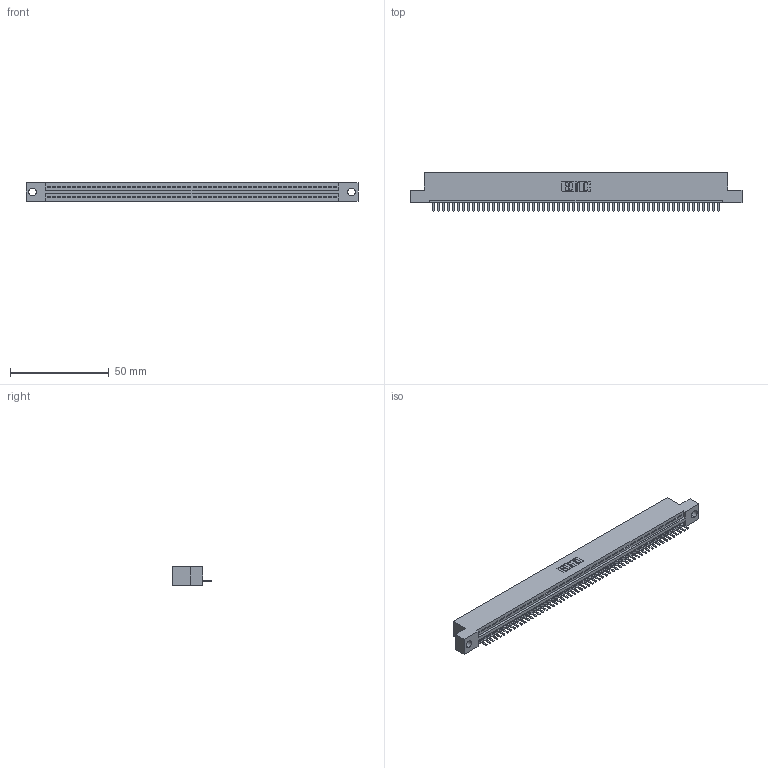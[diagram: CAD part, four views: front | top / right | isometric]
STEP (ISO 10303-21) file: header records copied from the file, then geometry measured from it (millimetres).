
FILE_DESCRIPTION (( 'STEP AP203' ), '1' );
FILE_NAME ('395-058-520-104.STEP', '2018-11-22T23:56:21', ( '' ), ( '' ), 'SwSTEP 2.0', 'SolidWorks 2016', '' );
FILE_SCHEMA (( 'CONFIG_CONTROL_DESIGN' ));
Length unit declared in the file: inch
Products named in the file (3): 345-292-001_345-293-120; 345 Part_Flush Mounting Lugs - 0.156 Dia-TH; 395-058-520-104
Assembly tree (59 placements, depth 2):
  395-058-520-104
    345 Part_Flush Mounting Lugs - 0.156 Dia-TH
    345-292-001_345-293-120  x58
Bounding box: 168.53 x 19.68 x 9.4 mm (x, y, z)
Volume: 15883.4 mm3; surface area: 20588 mm2
Topology: 59 solids, 59 shells, 3722 faces, 11013 edges, 7186 vertices
Faces by surface type: plane 2516, cylinder 1206
Entity records: 41615 total; most frequent: CARTESIAN_POINT 7226, ORIENTED_EDGE 7206, DIRECTION 6275, EDGE_CURVE 3603, VECTOR 3235, LINE 3235, VERTEX_POINT 2398, AXIS2_PLACEMENT_3D 1520
